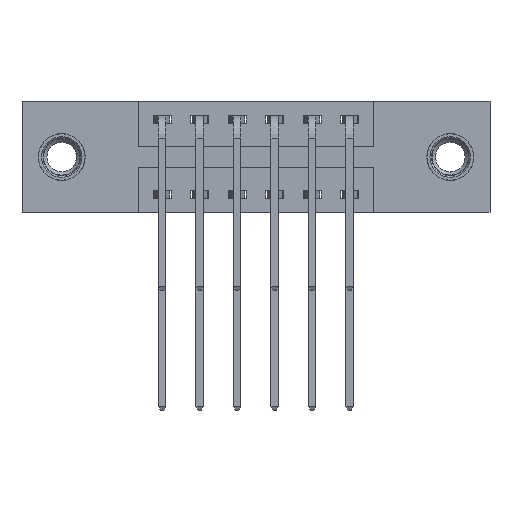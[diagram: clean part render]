
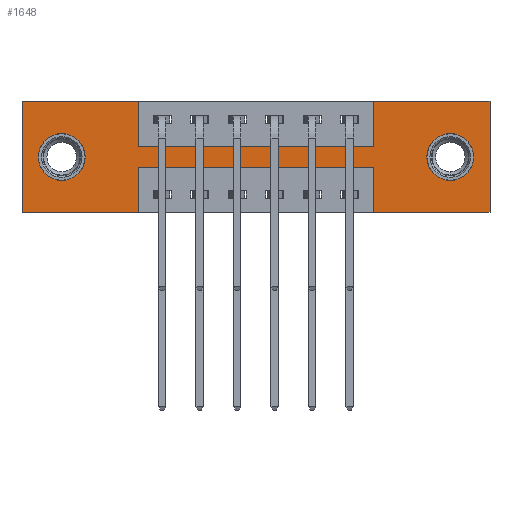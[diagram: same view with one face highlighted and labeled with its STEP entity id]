
A CAD part, front view. The second image highlights one B-rep face of the part: STEP entity #1648.
In plain terms, the highlighted planar face has unit normal (0, -1, 0).
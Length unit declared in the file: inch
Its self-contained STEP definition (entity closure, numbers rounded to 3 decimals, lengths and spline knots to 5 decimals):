
#120 = VERTEX_POINT ( 'NONE', #10430 ) ;
#159 = VERTEX_POINT ( 'NONE', #7185 ) ;
#189 = ORIENTED_EDGE ( 'NONE', *, *, #8461, .F. ) ;
#202 = DIRECTION ( 'NONE',  ( -1., 0., 0. ) ) ;
#339 = DIRECTION ( 'NONE',  ( 0., -1., 0. ) ) ;
#349 = EDGE_CURVE ( 'NONE', #3141, #120, #7402, .T. ) ;
#488 = VECTOR ( 'NONE', #8192, 39.37008 ) ;
#504 = CIRCLE ( 'NONE', #6896, 0.078 ) ;
#509 = DIRECTION ( 'NONE',  ( 0., 1., 0. ) ) ;
#683 = CARTESIAN_POINT ( 'NONE',  ( 0., 0., 0. ) ) ;
#699 = DIRECTION ( 'NONE',  ( 0., 1., 0. ) ) ;
#791 = ORIENTED_EDGE ( 'NONE', *, *, #9239, .F. ) ;
#803 = ORIENTED_EDGE ( 'NONE', *, *, #349, .F. ) ;
#832 = VECTOR ( 'NONE', #202, 39.37008 ) ;
#964 = CARTESIAN_POINT ( 'NONE',  ( 0.3875, 0., -0.15 ) ) ;
#969 = CARTESIAN_POINT ( 'NONE',  ( 0., 0., -0.37 ) ) ;
#998 = CARTESIAN_POINT ( 'NONE',  ( 1.56, 0., 0. ) ) ;
#1059 = CARTESIAN_POINT ( 'NONE',  ( 0.3875, 0., -0.37 ) ) ;
#1088 = VERTEX_POINT ( 'NONE', #10592 ) ;
#1185 = EDGE_CURVE ( 'NONE', #8761, #2490, #9961, .T. ) ;
#1257 = VERTEX_POINT ( 'NONE', #969 ) ;
#1304 = VECTOR ( 'NONE', #3069, 39.37008 ) ;
#1462 = CARTESIAN_POINT ( 'NONE',  ( 1.1725, 0., -0.37 ) ) ;
#1648 = ADVANCED_FACE ( 'NONE', ( #6103, #2849, #4971 ), #2137, .T. ) ;
#1816 = VECTOR ( 'NONE', #2539, 39.37008 ) ;
#1983 = CARTESIAN_POINT ( 'NONE',  ( 0.1325, 0., -0.185 ) ) ;
#2044 = ORIENTED_EDGE ( 'NONE', *, *, #5859, .F. ) ;
#2077 = AXIS2_PLACEMENT_3D ( 'NONE', #5800, #339, #7619 ) ;
#2137 = PLANE ( 'NONE',  #2077 ) ;
#2150 = CARTESIAN_POINT ( 'NONE',  ( 0.3875, 0., 0. ) ) ;
#2222 = VECTOR ( 'NONE', #11243, 39.37008 ) ;
#2297 = EDGE_LOOP ( 'NONE', ( #11263, #10347 ) ) ;
#2367 = ORIENTED_EDGE ( 'NONE', *, *, #1185, .F. ) ;
#2369 = DIRECTION ( 'NONE',  ( 0., 0., 1. ) ) ;
#2475 = DIRECTION ( 'NONE',  ( 1., 0., 0. ) ) ;
#2486 = VECTOR ( 'NONE', #2475, 39.37008 ) ;
#2490 = VERTEX_POINT ( 'NONE', #1059 ) ;
#2502 = LINE ( 'NONE', #2150, #7903 ) ;
#2539 = DIRECTION ( 'NONE',  ( 0., 0., 1. ) ) ;
#2689 = LINE ( 'NONE', #5667, #832 ) ;
#2724 = CARTESIAN_POINT ( 'NONE',  ( 0., 0., 0. ) ) ;
#2849 = FACE_BOUND ( 'NONE', #2297, .T. ) ;
#3015 = AXIS2_PLACEMENT_3D ( 'NONE', #10528, #509, #2369 ) ;
#3069 = DIRECTION ( 'NONE',  ( 1., 0., 0. ) ) ;
#3076 = VERTEX_POINT ( 'NONE', #964 ) ;
#3141 = VERTEX_POINT ( 'NONE', #8287 ) ;
#3401 = EDGE_CURVE ( 'NONE', #120, #6951, #8147, .T. ) ;
#3422 = DIRECTION ( 'NONE',  ( 0., 0., -1. ) ) ;
#3466 = CARTESIAN_POINT ( 'NONE',  ( 0.1325, 0., -0.107 ) ) ;
#3644 = EDGE_CURVE ( 'NONE', #6248, #11123, #7476, .T. ) ;
#3684 = CARTESIAN_POINT ( 'NONE',  ( 1.4275, 0., -0.107 ) ) ;
#3701 = VECTOR ( 'NONE', #3846, 39.37008 ) ;
#3783 = CARTESIAN_POINT ( 'NONE',  ( 0.3875, 0., -0.22 ) ) ;
#3846 = DIRECTION ( 'NONE',  ( -1., 0., 0. ) ) ;
#3983 = EDGE_CURVE ( 'NONE', #5707, #9883, #7134, .T. ) ;
#3998 = EDGE_CURVE ( 'NONE', #2490, #1257, #10924, .T. ) ;
#4016 = VECTOR ( 'NONE', #11360, 39.37008 ) ;
#4099 = LINE ( 'NONE', #9423, #1304 ) ;
#4160 = CARTESIAN_POINT ( 'NONE',  ( 1.1725, 0., 0. ) ) ;
#4250 = CIRCLE ( 'NONE', #5813, 0.078 ) ;
#4587 = LINE ( 'NONE', #683, #2486 ) ;
#4799 = CARTESIAN_POINT ( 'NONE',  ( 1.4275, 0., -0.185 ) ) ;
#4971 = FACE_OUTER_BOUND ( 'NONE', #7775, .T. ) ;
#5134 = EDGE_CURVE ( 'NONE', #9908, #8761, #2689, .T. ) ;
#5142 = VECTOR ( 'NONE', #3422, 39.37008 ) ;
#5559 = CARTESIAN_POINT ( 'NONE',  ( 1.56, 0., -0.37 ) ) ;
#5626 = LINE ( 'NONE', #4160, #4016 ) ;
#5648 = DIRECTION ( 'NONE',  ( 0., 0., 1. ) ) ;
#5667 = CARTESIAN_POINT ( 'NONE',  ( 0.3875, 0., -0.22 ) ) ;
#5707 = VERTEX_POINT ( 'NONE', #5722 ) ;
#5715 = DIRECTION ( 'NONE',  ( 0., 1., 0. ) ) ;
#5722 = CARTESIAN_POINT ( 'NONE',  ( 1.4275, 0., -0.263 ) ) ;
#5739 = VECTOR ( 'NONE', #7350, 39.37008 ) ;
#5744 = CARTESIAN_POINT ( 'NONE',  ( 0., 0., -0.37 ) ) ;
#5800 = CARTESIAN_POINT ( 'NONE',  ( 0., 0., -0.37 ) ) ;
#5813 = AXIS2_PLACEMENT_3D ( 'NONE', #1983, #5715, #5648 ) ;
#5858 = EDGE_CURVE ( 'NONE', #159, #3076, #2502, .T. ) ;
#5859 = EDGE_CURVE ( 'NONE', #6951, #11364, #11278, .T. ) ;
#5915 = ORIENTED_EDGE ( 'NONE', *, *, #5858, .F. ) ;
#6103 = FACE_BOUND ( 'NONE', #11664, .T. ) ;
#6106 = EDGE_CURVE ( 'NONE', #1088, #159, #4587, .T. ) ;
#6248 = VERTEX_POINT ( 'NONE', #3466 ) ;
#6488 = CARTESIAN_POINT ( 'NONE',  ( 1.1725, 0., -0.22 ) ) ;
#6896 = AXIS2_PLACEMENT_3D ( 'NONE', #9676, #699, #11506 ) ;
#6951 = VERTEX_POINT ( 'NONE', #5559 ) ;
#6988 = VERTEX_POINT ( 'NONE', #7542 ) ;
#6992 = ORIENTED_EDGE ( 'NONE', *, *, #3998, .F. ) ;
#7134 = CIRCLE ( 'NONE', #9620, 0.078 ) ;
#7185 = CARTESIAN_POINT ( 'NONE',  ( 0.3875, 0., 0. ) ) ;
#7208 = LINE ( 'NONE', #1462, #1816 ) ;
#7350 = DIRECTION ( 'NONE',  ( 0., 0., -1. ) ) ;
#7361 = EDGE_CURVE ( 'NONE', #1257, #1088, #8975, .T. ) ;
#7402 = LINE ( 'NONE', #10679, #7684 ) ;
#7457 = DIRECTION ( 'NONE',  ( 0., 0., -1. ) ) ;
#7476 = CIRCLE ( 'NONE', #3015, 0.078 ) ;
#7542 = CARTESIAN_POINT ( 'NONE',  ( 1.1725, 0., -0.15 ) ) ;
#7619 = DIRECTION ( 'NONE',  ( 0., 0., -1. ) ) ;
#7684 = VECTOR ( 'NONE', #11572, 39.37008 ) ;
#7775 = EDGE_LOOP ( 'NONE', ( #2367, #8866, #791, #2044, #9299, #803, #8042, #189, #5915, #8974, #9071, #6992 ) ) ;
#7903 = VECTOR ( 'NONE', #8462, 39.37008 ) ;
#8042 = ORIENTED_EDGE ( 'NONE', *, *, #10317, .F. ) ;
#8065 = CARTESIAN_POINT ( 'NONE',  ( 0.3875, 0., -0.37 ) ) ;
#8147 = LINE ( 'NONE', #998, #5739 ) ;
#8192 = DIRECTION ( 'NONE',  ( 0., 0., 1. ) ) ;
#8220 = EDGE_CURVE ( 'NONE', #11123, #6248, #4250, .T. ) ;
#8287 = CARTESIAN_POINT ( 'NONE',  ( 1.1725, 0., 0. ) ) ;
#8461 = EDGE_CURVE ( 'NONE', #3076, #6988, #4099, .T. ) ;
#8462 = DIRECTION ( 'NONE',  ( 0., 0., -1. ) ) ;
#8496 = CARTESIAN_POINT ( 'NONE',  ( 0., 0., -0.37 ) ) ;
#8761 = VERTEX_POINT ( 'NONE', #3783 ) ;
#8866 = ORIENTED_EDGE ( 'NONE', *, *, #5134, .F. ) ;
#8974 = ORIENTED_EDGE ( 'NONE', *, *, #6106, .F. ) ;
#8975 = LINE ( 'NONE', #2724, #488 ) ;
#8995 = ORIENTED_EDGE ( 'NONE', *, *, #9949, .T. ) ;
#9070 = ORIENTED_EDGE ( 'NONE', *, *, #3983, .T. ) ;
#9071 = ORIENTED_EDGE ( 'NONE', *, *, #7361, .F. ) ;
#9225 = CARTESIAN_POINT ( 'NONE',  ( 1.1725, 0., -0.37 ) ) ;
#9239 = EDGE_CURVE ( 'NONE', #11364, #9908, #7208, .T. ) ;
#9299 = ORIENTED_EDGE ( 'NONE', *, *, #3401, .F. ) ;
#9423 = CARTESIAN_POINT ( 'NONE',  ( 0.3875, 0., -0.15 ) ) ;
#9620 = AXIS2_PLACEMENT_3D ( 'NONE', #4799, #11150, #7457 ) ;
#9676 = CARTESIAN_POINT ( 'NONE',  ( 1.4275, 0., -0.185 ) ) ;
#9883 = VERTEX_POINT ( 'NONE', #3684 ) ;
#9908 = VERTEX_POINT ( 'NONE', #6488 ) ;
#9949 = EDGE_CURVE ( 'NONE', #9883, #5707, #504, .T. ) ;
#9961 = LINE ( 'NONE', #8065, #5142 ) ;
#10317 = EDGE_CURVE ( 'NONE', #6988, #3141, #5626, .T. ) ;
#10347 = ORIENTED_EDGE ( 'NONE', *, *, #8220, .T. ) ;
#10430 = CARTESIAN_POINT ( 'NONE',  ( 1.56, 0., 0. ) ) ;
#10528 = CARTESIAN_POINT ( 'NONE',  ( 0.1325, 0., -0.185 ) ) ;
#10542 = CARTESIAN_POINT ( 'NONE',  ( 0.1325, 0., -0.263 ) ) ;
#10592 = CARTESIAN_POINT ( 'NONE',  ( 0., 0., 0. ) ) ;
#10679 = CARTESIAN_POINT ( 'NONE',  ( 0., 0., 0. ) ) ;
#10924 = LINE ( 'NONE', #5744, #3701 ) ;
#11123 = VERTEX_POINT ( 'NONE', #10542 ) ;
#11150 = DIRECTION ( 'NONE',  ( 0., 1., 0. ) ) ;
#11243 = DIRECTION ( 'NONE',  ( -1., 0., 0. ) ) ;
#11263 = ORIENTED_EDGE ( 'NONE', *, *, #3644, .T. ) ;
#11278 = LINE ( 'NONE', #8496, #2222 ) ;
#11360 = DIRECTION ( 'NONE',  ( 0., 0., 1. ) ) ;
#11364 = VERTEX_POINT ( 'NONE', #9225 ) ;
#11506 = DIRECTION ( 'NONE',  ( 0., 0., -1. ) ) ;
#11572 = DIRECTION ( 'NONE',  ( 1., 0., 0. ) ) ;
#11664 = EDGE_LOOP ( 'NONE', ( #8995, #9070 ) ) ;
